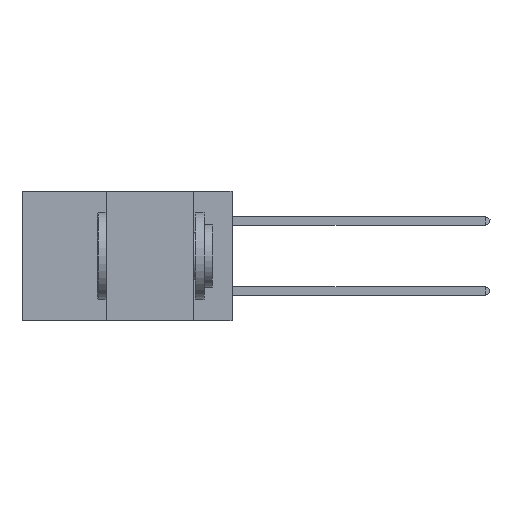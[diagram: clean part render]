
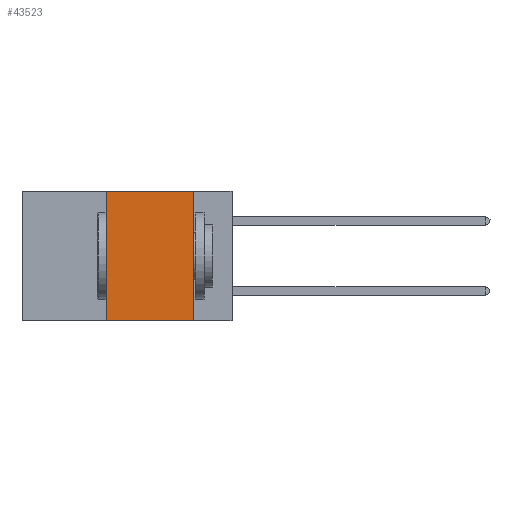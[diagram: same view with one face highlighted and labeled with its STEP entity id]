
A CAD part, left-side view. The second image highlights one B-rep face of the part: STEP entity #43523.
In plain terms, the highlighted planar face has unit normal (-1, 0, 0).
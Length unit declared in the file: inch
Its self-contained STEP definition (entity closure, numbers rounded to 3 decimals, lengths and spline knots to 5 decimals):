
#284 = VERTEX_POINT ( 'NONE', #27943 ) ;
#1146 = CARTESIAN_POINT ( 'NONE',  ( 0., 0.11, 0. ) ) ;
#2069 = DIRECTION ( 'NONE',  ( 1., 0., 0. ) ) ;
#2376 = FACE_OUTER_BOUND ( 'NONE', #12349, .T. ) ;
#3565 = ORIENTED_EDGE ( 'NONE', *, *, #38795, .F. ) ;
#4366 = AXIS2_PLACEMENT_3D ( 'NONE', #9377, #2069, #27458 ) ;
#4894 = VECTOR ( 'NONE', #10140, 39.37008 ) ;
#6609 = VERTEX_POINT ( 'NONE', #18296 ) ;
#6669 = DIRECTION ( 'NONE',  ( 0., 0., -1. ) ) ;
#8627 = CARTESIAN_POINT ( 'NONE',  ( 0., 0.36, 0. ) ) ;
#9377 = CARTESIAN_POINT ( 'NONE',  ( 0., 0.6, 0. ) ) ;
#10140 = DIRECTION ( 'NONE',  ( 0., -1., 0. ) ) ;
#10353 = VERTEX_POINT ( 'NONE', #8627 ) ;
#12349 = EDGE_LOOP ( 'NONE', ( #28732, #35302, #3565, #37655 ) ) ;
#12794 = DIRECTION ( 'NONE',  ( 0., 0., 1. ) ) ;
#13690 = LINE ( 'NONE', #34004, #40561 ) ;
#14638 = LINE ( 'NONE', #28263, #33471 ) ;
#15899 = DIRECTION ( 'NONE',  ( 0., -1., 0. ) ) ;
#18296 = CARTESIAN_POINT ( 'NONE',  ( 0., 0.36, -0.37 ) ) ;
#21350 = VERTEX_POINT ( 'NONE', #1146 ) ;
#23025 = LINE ( 'NONE', #33510, #41479 ) ;
#27458 = DIRECTION ( 'NONE',  ( 0., 0., -1. ) ) ;
#27943 = CARTESIAN_POINT ( 'NONE',  ( 0., 0.11, -0.37 ) ) ;
#28037 = CARTESIAN_POINT ( 'NONE',  ( 0., 0.6, -0.37 ) ) ;
#28263 = CARTESIAN_POINT ( 'NONE',  ( 0., 0.11, 0. ) ) ;
#28732 = ORIENTED_EDGE ( 'NONE', *, *, #41067, .F. ) ;
#33471 = VECTOR ( 'NONE', #6669, 39.37008 ) ;
#33510 = CARTESIAN_POINT ( 'NONE',  ( 0., 0.6, 0. ) ) ;
#34004 = CARTESIAN_POINT ( 'NONE',  ( 0., 0.36, 0. ) ) ;
#34202 = EDGE_CURVE ( 'NONE', #6609, #284, #42608, .T. ) ;
#35154 = EDGE_CURVE ( 'NONE', #10353, #21350, #23025, .T. ) ;
#35302 = ORIENTED_EDGE ( 'NONE', *, *, #35154, .F. ) ;
#37655 = ORIENTED_EDGE ( 'NONE', *, *, #34202, .T. ) ;
#38795 = EDGE_CURVE ( 'NONE', #6609, #10353, #13690, .T. ) ;
#40561 = VECTOR ( 'NONE', #12794, 39.37008 ) ;
#41067 = EDGE_CURVE ( 'NONE', #21350, #284, #14638, .T. ) ;
#41479 = VECTOR ( 'NONE', #15899, 39.37008 ) ;
#42608 = LINE ( 'NONE', #28037, #4894 ) ;
#43523 = ADVANCED_FACE ( 'NONE', ( #2376 ), #44592, .F. ) ;
#44592 = PLANE ( 'NONE',  #4366 ) ;
